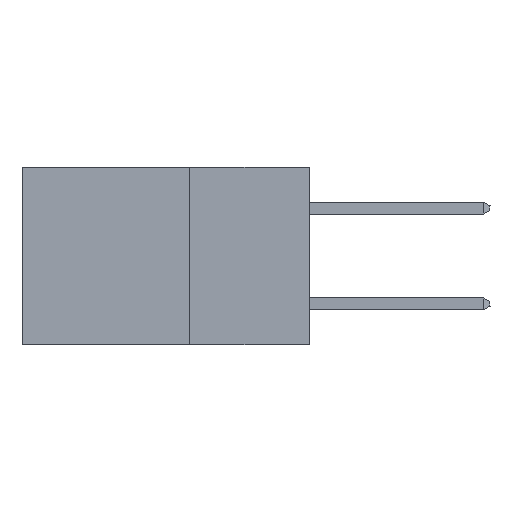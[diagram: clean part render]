
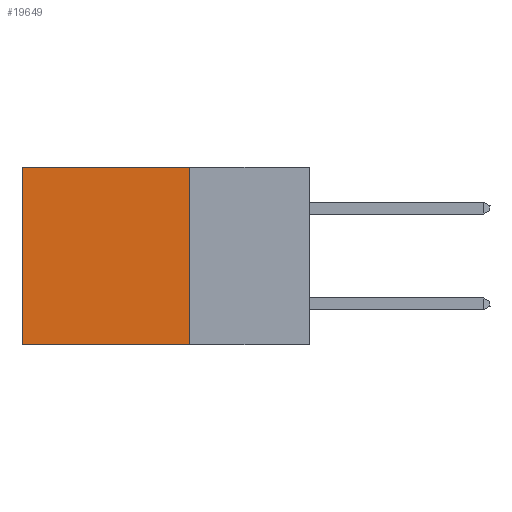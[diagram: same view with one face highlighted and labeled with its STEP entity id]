
A CAD part, left-side view. The second image highlights one B-rep face of the part: STEP entity #19649.
In plain terms, the highlighted planar face has unit normal (-1, 0, 0).
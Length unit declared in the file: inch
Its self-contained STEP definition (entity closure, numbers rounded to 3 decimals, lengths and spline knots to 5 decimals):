
#1674 = LINE ( 'NONE', #8062, #21270 ) ;
#2651 = CARTESIAN_POINT ( 'NONE',  ( 0.2875, 0.6, 0. ) ) ;
#3292 = AXIS2_PLACEMENT_3D ( 'NONE', #18848, #19005, #18930 ) ;
#3592 = EDGE_CURVE ( 'NONE', #21376, #10135, #4786, .T. ) ;
#4028 = PLANE ( 'NONE',  #3292 ) ;
#4786 = LINE ( 'NONE', #2651, #12568 ) ;
#5088 = DIRECTION ( 'NONE',  ( 0., 1., 0. ) ) ;
#5877 = CARTESIAN_POINT ( 'NONE',  ( 0.2875, 0.6, 0. ) ) ;
#7067 = CARTESIAN_POINT ( 'NONE',  ( 0.2875, 0.25, 0. ) ) ;
#7188 = CARTESIAN_POINT ( 'NONE',  ( 0.2875, 0.6, -0.37 ) ) ;
#7225 = ORIENTED_EDGE ( 'NONE', *, *, #3592, .T. ) ;
#7226 = CARTESIAN_POINT ( 'NONE',  ( 0.2875, 0.25, -0.37 ) ) ;
#8062 = CARTESIAN_POINT ( 'NONE',  ( 0.2875, 0.25, 0. ) ) ;
#8145 = FACE_OUTER_BOUND ( 'NONE', #15536, .T. ) ;
#9117 = CARTESIAN_POINT ( 'NONE',  ( 0.2875, 0.25, 0. ) ) ;
#9464 = ORIENTED_EDGE ( 'NONE', *, *, #19962, .F. ) ;
#9952 = VECTOR ( 'NONE', #5088, 39.37008 ) ;
#10135 = VERTEX_POINT ( 'NONE', #7188 ) ;
#12568 = VECTOR ( 'NONE', #17411, 39.37008 ) ;
#13376 = EDGE_CURVE ( 'NONE', #21426, #19869, #1674, .T. ) ;
#13528 = ORIENTED_EDGE ( 'NONE', *, *, #13376, .F. ) ;
#13668 = LINE ( 'NONE', #7067, #9952 ) ;
#15536 = EDGE_LOOP ( 'NONE', ( #7225, #9464, #13528, #16262 ) ) ;
#16262 = ORIENTED_EDGE ( 'NONE', *, *, #22874, .T. ) ;
#17004 = DIRECTION ( 'NONE',  ( 0., 1., 0. ) ) ;
#17411 = DIRECTION ( 'NONE',  ( 0., 0., -1. ) ) ;
#17555 = DIRECTION ( 'NONE',  ( 0., 0., -1. ) ) ;
#18482 = LINE ( 'NONE', #20961, #19045 ) ;
#18848 = CARTESIAN_POINT ( 'NONE',  ( 0.2875, 0.25, 0. ) ) ;
#18930 = DIRECTION ( 'NONE',  ( 0., 0., -1. ) ) ;
#19005 = DIRECTION ( 'NONE',  ( 1., 0., 0. ) ) ;
#19045 = VECTOR ( 'NONE', #17004, 39.37008 ) ;
#19649 = ADVANCED_FACE ( 'NONE', ( #8145 ), #4028, .F. ) ;
#19869 = VERTEX_POINT ( 'NONE', #7226 ) ;
#19962 = EDGE_CURVE ( 'NONE', #19869, #10135, #18482, .T. ) ;
#20961 = CARTESIAN_POINT ( 'NONE',  ( 0.2875, 0.25, -0.37 ) ) ;
#21270 = VECTOR ( 'NONE', #17555, 39.37008 ) ;
#21376 = VERTEX_POINT ( 'NONE', #5877 ) ;
#21426 = VERTEX_POINT ( 'NONE', #9117 ) ;
#22874 = EDGE_CURVE ( 'NONE', #21426, #21376, #13668, .T. ) ;
